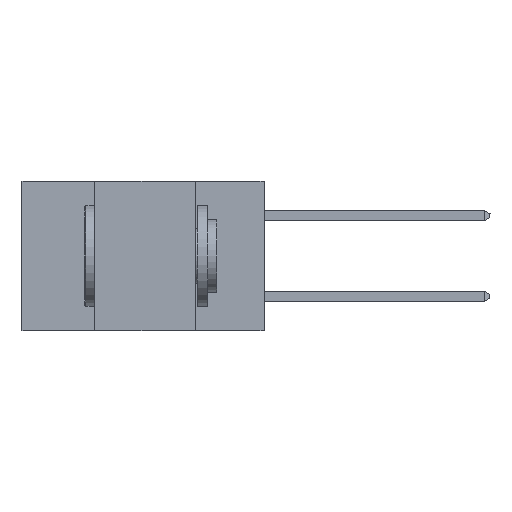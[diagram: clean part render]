
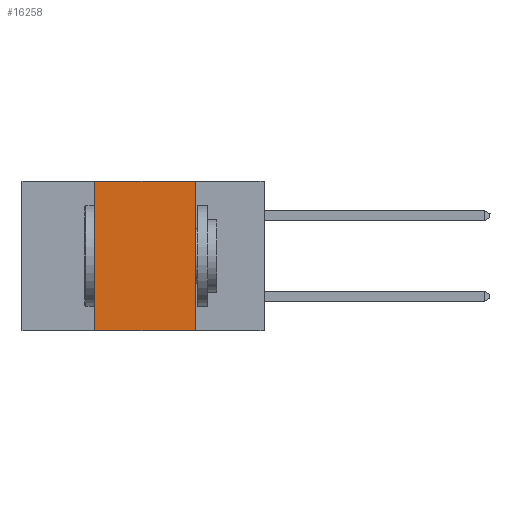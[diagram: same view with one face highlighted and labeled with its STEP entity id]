
A CAD part, left-side view. The second image highlights one B-rep face of the part: STEP entity #16258.
In plain terms, the highlighted planar face has unit normal (-1, 0, 0).
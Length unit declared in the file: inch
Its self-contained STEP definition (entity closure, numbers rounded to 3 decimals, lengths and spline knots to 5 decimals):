
#890 = DIRECTION ( 'NONE',  ( 0., 0., -1. ) ) ;
#927 = CARTESIAN_POINT ( 'NONE',  ( 0., 0.42, 0. ) ) ;
#2071 = VECTOR ( 'NONE', #5040, 39.37008 ) ;
#2076 = CARTESIAN_POINT ( 'NONE',  ( 0., 0.17, 0. ) ) ;
#2099 = ORIENTED_EDGE ( 'NONE', *, *, #23984, .F. ) ;
#3318 = VECTOR ( 'NONE', #19180, 39.37008 ) ;
#5040 = DIRECTION ( 'NONE',  ( 0., 0., 1. ) ) ;
#6494 = CARTESIAN_POINT ( 'NONE',  ( 0., 0.6, 0. ) ) ;
#6932 = EDGE_CURVE ( 'NONE', #19137, #15938, #24083, .T. ) ;
#7439 = AXIS2_PLACEMENT_3D ( 'NONE', #6494, #19599, #12159 ) ;
#7860 = VECTOR ( 'NONE', #10473, 39.37008 ) ;
#9333 = CARTESIAN_POINT ( 'NONE',  ( 0., 0.42, -0.37 ) ) ;
#10145 = ORIENTED_EDGE ( 'NONE', *, *, #6932, .F. ) ;
#10473 = DIRECTION ( 'NONE',  ( 0., -1., 0. ) ) ;
#10604 = EDGE_CURVE ( 'NONE', #13940, #11580, #23565, .T. ) ;
#11580 = VERTEX_POINT ( 'NONE', #22237 ) ;
#12159 = DIRECTION ( 'NONE',  ( 0., 0., -1. ) ) ;
#13940 = VERTEX_POINT ( 'NONE', #22586 ) ;
#14618 = LINE ( 'NONE', #19790, #7860 ) ;
#15601 = FACE_OUTER_BOUND ( 'NONE', #20691, .T. ) ;
#15938 = VERTEX_POINT ( 'NONE', #927 ) ;
#16044 = PLANE ( 'NONE',  #7439 ) ;
#16258 = ADVANCED_FACE ( 'NONE', ( #15601 ), #16044, .F. ) ;
#17120 = LINE ( 'NONE', #23226, #3318 ) ;
#17306 = ORIENTED_EDGE ( 'NONE', *, *, #18005, .T. ) ;
#18005 = EDGE_CURVE ( 'NONE', #19137, #11580, #14618, .T. ) ;
#18066 = CARTESIAN_POINT ( 'NONE',  ( 0., 0.42, 0. ) ) ;
#18532 = VECTOR ( 'NONE', #890, 39.37008 ) ;
#19137 = VERTEX_POINT ( 'NONE', #9333 ) ;
#19180 = DIRECTION ( 'NONE',  ( 0., -1., 0. ) ) ;
#19599 = DIRECTION ( 'NONE',  ( 1., 0., 0. ) ) ;
#19790 = CARTESIAN_POINT ( 'NONE',  ( 0., 0.6, -0.37 ) ) ;
#20691 = EDGE_LOOP ( 'NONE', ( #22895, #2099, #10145, #17306 ) ) ;
#22237 = CARTESIAN_POINT ( 'NONE',  ( 0., 0.17, -0.37 ) ) ;
#22586 = CARTESIAN_POINT ( 'NONE',  ( 0., 0.17, 0. ) ) ;
#22895 = ORIENTED_EDGE ( 'NONE', *, *, #10604, .F. ) ;
#23226 = CARTESIAN_POINT ( 'NONE',  ( 0., 0.6, 0. ) ) ;
#23565 = LINE ( 'NONE', #2076, #18532 ) ;
#23984 = EDGE_CURVE ( 'NONE', #15938, #13940, #17120, .T. ) ;
#24083 = LINE ( 'NONE', #18066, #2071 ) ;
